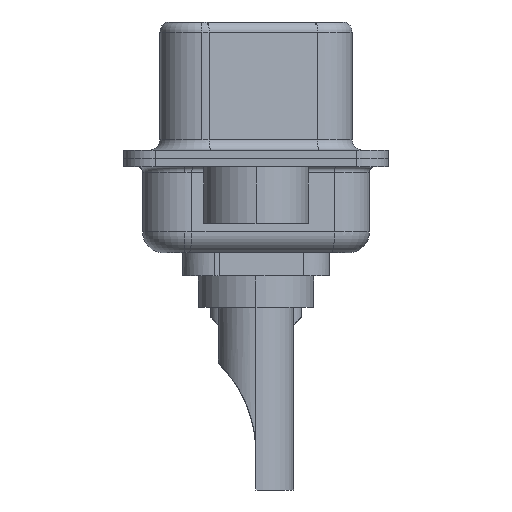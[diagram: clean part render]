
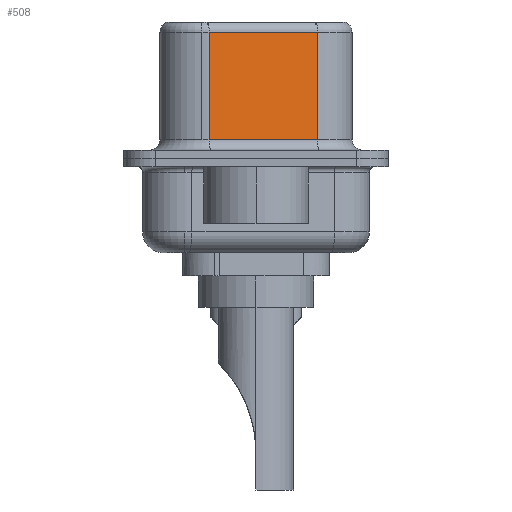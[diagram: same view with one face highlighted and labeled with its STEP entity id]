
A CAD part, left-side view. The second image highlights one B-rep face of the part: STEP entity #508.
In plain terms, the highlighted planar face has unit normal (-0.985, -0.174, 0).
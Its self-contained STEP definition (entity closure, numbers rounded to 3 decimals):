
#176 = CARTESIAN_POINT ( 'NONE',  ( 4.58, -2.927, 6.52 ) ) ;
#508 = ADVANCED_FACE ( 'NONE', ( #1984 ), #10538, .F. ) ;
#854 = ORIENTED_EDGE ( 'NONE', *, *, #13862, .T. ) ;
#982 = DIRECTION ( 'NONE',  ( 0., 0., -1. ) ) ;
#1298 = CARTESIAN_POINT ( 'NONE',  ( 4.58, -2.927, 6.02 ) ) ;
#1984 = FACE_OUTER_BOUND ( 'NONE', #6642, .T. ) ;
#3867 = CARTESIAN_POINT ( 'NONE',  ( 3.67, 2.233, 6.02 ) ) ;
#5219 = ORIENTED_EDGE ( 'NONE', *, *, #17512, .T. ) ;
#5867 = CARTESIAN_POINT ( 'NONE',  ( 3.67, 2.233, 0.9 ) ) ;
#6623 = ORIENTED_EDGE ( 'NONE', *, *, #11898, .T. ) ;
#6642 = EDGE_LOOP ( 'NONE', ( #11366, #854, #6623, #5219 ) ) ;
#7609 = VECTOR ( 'NONE', #982, 1000. ) ;
#9853 = VECTOR ( 'NONE', #15825, 1000. ) ;
#10428 = LINE ( 'NONE', #1298, #9853 ) ;
#10538 = PLANE ( 'NONE',  #19835 ) ;
#10548 = DIRECTION ( 'NONE',  ( 0.174, -0.985, 0. ) ) ;
#10975 = VERTEX_POINT ( 'NONE', #3867 ) ;
#11040 = VERTEX_POINT ( 'NONE', #5867 ) ;
#11333 = LINE ( 'NONE', #13694, #7609 ) ;
#11366 = ORIENTED_EDGE ( 'NONE', *, *, #19954, .F. ) ;
#11898 = EDGE_CURVE ( 'NONE', #10975, #11040, #11333, .T. ) ;
#12974 = DIRECTION ( 'NONE',  ( -0.174, 0.985, 0. ) ) ;
#13694 = CARTESIAN_POINT ( 'NONE',  ( 3.67, 2.233, 6.52 ) ) ;
#13862 = EDGE_CURVE ( 'NONE', #20848, #10975, #10428, .T. ) ;
#14403 = DIRECTION ( 'NONE',  ( 0., 0., -1. ) ) ;
#15825 = DIRECTION ( 'NONE',  ( -0.174, 0.985, 0. ) ) ;
#15849 = CARTESIAN_POINT ( 'NONE',  ( 4.58, -2.927, 6.02 ) ) ;
#16433 = LINE ( 'NONE', #23279, #17583 ) ;
#16807 = DIRECTION ( 'NONE',  ( 0.985, 0.174, 0. ) ) ;
#17512 = EDGE_CURVE ( 'NONE', #11040, #17991, #16433, .T. ) ;
#17583 = VECTOR ( 'NONE', #10548, 1000. ) ;
#17991 = VERTEX_POINT ( 'NONE', #19183 ) ;
#18072 = CARTESIAN_POINT ( 'NONE',  ( 4.58, -2.927, 6.52 ) ) ;
#19183 = CARTESIAN_POINT ( 'NONE',  ( 4.58, -2.927, 0.9 ) ) ;
#19835 = AXIS2_PLACEMENT_3D ( 'NONE', #176, #16807, #12974 ) ;
#19954 = EDGE_CURVE ( 'NONE', #20848, #17991, #22878, .T. ) ;
#20848 = VERTEX_POINT ( 'NONE', #15849 ) ;
#21754 = VECTOR ( 'NONE', #14403, 1000. ) ;
#22878 = LINE ( 'NONE', #18072, #21754 ) ;
#23279 = CARTESIAN_POINT ( 'NONE',  ( 4.58, -2.927, 0.9 ) ) ;
